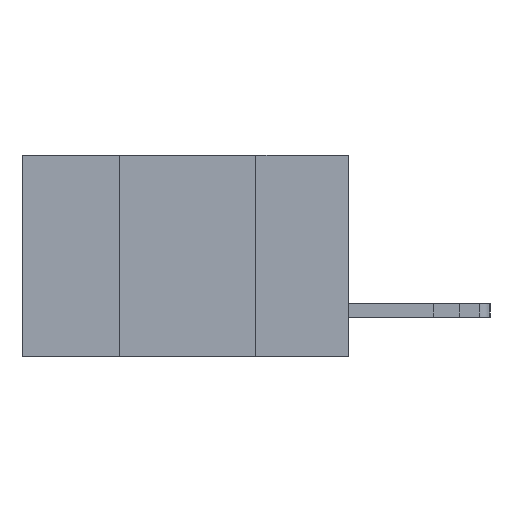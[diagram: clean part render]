
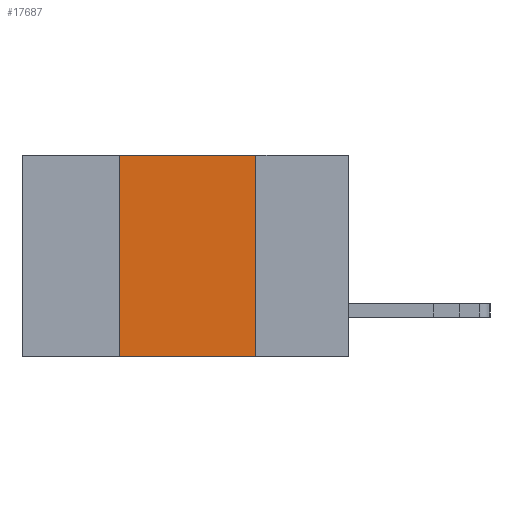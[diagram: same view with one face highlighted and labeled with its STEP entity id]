
A CAD part, left-side view. The second image highlights one B-rep face of the part: STEP entity #17687.
In plain terms, the highlighted planar face has unit normal (-1, 0, 0).
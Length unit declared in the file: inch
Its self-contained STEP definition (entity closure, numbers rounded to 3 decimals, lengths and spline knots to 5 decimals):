
#396 = VERTEX_POINT ( 'NONE', #24051 ) ;
#1382 = LINE ( 'NONE', #6650, #16343 ) ;
#1597 = LINE ( 'NONE', #7214, #17160 ) ;
#1677 = EDGE_CURVE ( 'NONE', #15218, #396, #1597, .T. ) ;
#3112 = AXIS2_PLACEMENT_3D ( 'NONE', #17013, #4865, #19045 ) ;
#4810 = ORIENTED_EDGE ( 'NONE', *, *, #25158, .T. ) ;
#4865 = DIRECTION ( 'NONE',  ( 1., 0., 0. ) ) ;
#5945 = VERTEX_POINT ( 'NONE', #12689 ) ;
#5992 = ORIENTED_EDGE ( 'NONE', *, *, #16998, .F. ) ;
#6299 = LINE ( 'NONE', #20536, #16498 ) ;
#6558 = DIRECTION ( 'NONE',  ( 0., -1., 0. ) ) ;
#6650 = CARTESIAN_POINT ( 'NONE',  ( 0., 0.6, 0. ) ) ;
#7214 = CARTESIAN_POINT ( 'NONE',  ( 0., 0.17, 0. ) ) ;
#7702 = ORIENTED_EDGE ( 'NONE', *, *, #1677, .F. ) ;
#8016 = DIRECTION ( 'NONE',  ( 0., -1., 0. ) ) ;
#8288 = DIRECTION ( 'NONE',  ( 0., 0., 1. ) ) ;
#11768 = EDGE_LOOP ( 'NONE', ( #7702, #5992, #23017, #4810 ) ) ;
#12491 = DIRECTION ( 'NONE',  ( 0., 0., -1. ) ) ;
#12662 = VECTOR ( 'NONE', #8016, 39.37008 ) ;
#12689 = CARTESIAN_POINT ( 'NONE',  ( 0., 0.42, -0.37 ) ) ;
#12934 = PLANE ( 'NONE',  #3112 ) ;
#15218 = VERTEX_POINT ( 'NONE', #23835 ) ;
#16343 = VECTOR ( 'NONE', #6558, 39.37008 ) ;
#16498 = VECTOR ( 'NONE', #8288, 39.37008 ) ;
#16998 = EDGE_CURVE ( 'NONE', #18050, #15218, #1382, .T. ) ;
#17013 = CARTESIAN_POINT ( 'NONE',  ( 0., 0.6, 0. ) ) ;
#17160 = VECTOR ( 'NONE', #12491, 39.37008 ) ;
#17687 = ADVANCED_FACE ( 'NONE', ( #19452 ), #12934, .F. ) ;
#18050 = VERTEX_POINT ( 'NONE', #26108 ) ;
#18070 = LINE ( 'NONE', #26173, #12662 ) ;
#19045 = DIRECTION ( 'NONE',  ( 0., 0., -1. ) ) ;
#19452 = FACE_OUTER_BOUND ( 'NONE', #11768, .T. ) ;
#19564 = EDGE_CURVE ( 'NONE', #5945, #18050, #6299, .T. ) ;
#20536 = CARTESIAN_POINT ( 'NONE',  ( 0., 0.42, 0. ) ) ;
#23017 = ORIENTED_EDGE ( 'NONE', *, *, #19564, .F. ) ;
#23835 = CARTESIAN_POINT ( 'NONE',  ( 0., 0.17, 0. ) ) ;
#24051 = CARTESIAN_POINT ( 'NONE',  ( 0., 0.17, -0.37 ) ) ;
#25158 = EDGE_CURVE ( 'NONE', #5945, #396, #18070, .T. ) ;
#26108 = CARTESIAN_POINT ( 'NONE',  ( 0., 0.42, 0. ) ) ;
#26173 = CARTESIAN_POINT ( 'NONE',  ( 0., 0.6, -0.37 ) ) ;
